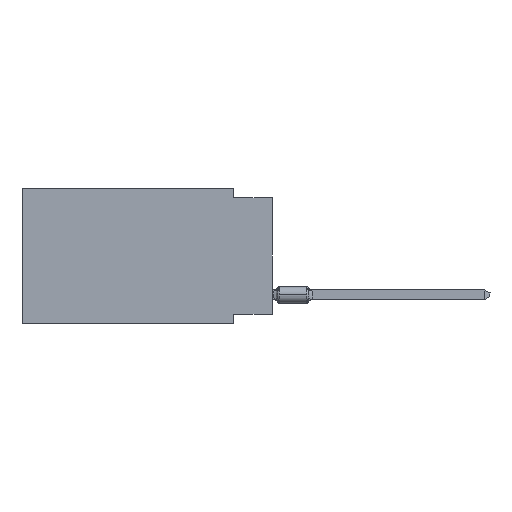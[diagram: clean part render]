
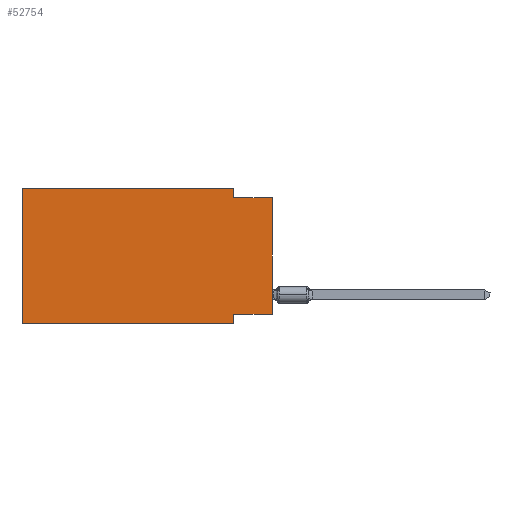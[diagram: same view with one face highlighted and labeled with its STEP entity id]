
A CAD part, left-side view. The second image highlights one B-rep face of the part: STEP entity #52754.
In plain terms, the highlighted planar face has unit normal (-1, 0, 0).
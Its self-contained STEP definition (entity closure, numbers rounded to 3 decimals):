
#568 = PLANE ( 'NONE',  #59043 ) ;
#885 = CARTESIAN_POINT ( 'NONE',  ( 0., 16.383, -8.89 ) ) ;
#1793 = DIRECTION ( 'NONE',  ( 0., 0., 1. ) ) ;
#2591 = CARTESIAN_POINT ( 'NONE',  ( 0., 2.54, -8.89 ) ) ;
#4227 = VERTEX_POINT ( 'NONE', #55370 ) ;
#4961 = CARTESIAN_POINT ( 'NONE',  ( 0., 0., -0.635 ) ) ;
#8224 = VECTOR ( 'NONE', #14936, 1000. ) ;
#10448 = LINE ( 'NONE', #34493, #51431 ) ;
#10690 = CARTESIAN_POINT ( 'NONE',  ( 0., 16.383, 0. ) ) ;
#11004 = VECTOR ( 'NONE', #1793, 1000. ) ;
#12177 = EDGE_CURVE ( 'NONE', #58907, #16448, #28717, .T. ) ;
#13767 = EDGE_CURVE ( 'NONE', #4227, #40827, #45387, .T. ) ;
#14033 = DIRECTION ( 'NONE',  ( 0., 0., -1. ) ) ;
#14936 = DIRECTION ( 'NONE',  ( 0., 1., 0. ) ) ;
#14949 = CARTESIAN_POINT ( 'NONE',  ( 0., 2.54, 0. ) ) ;
#15341 = EDGE_CURVE ( 'NONE', #35343, #16448, #57782, .T. ) ;
#16448 = VERTEX_POINT ( 'NONE', #4961 ) ;
#17211 = VERTEX_POINT ( 'NONE', #45778 ) ;
#18055 = ORIENTED_EDGE ( 'NONE', *, *, #25695, .F. ) ;
#20013 = VERTEX_POINT ( 'NONE', #10690 ) ;
#20449 = EDGE_LOOP ( 'NONE', ( #37459, #60444, #48436, #32620, #18055, #57352, #57975, #26336 ) ) ;
#21483 = LINE ( 'NONE', #26184, #60625 ) ;
#21529 = VECTOR ( 'NONE', #24655, 1000. ) ;
#24655 = DIRECTION ( 'NONE',  ( 0., -1., 0. ) ) ;
#25243 = DIRECTION ( 'NONE',  ( 1., 0., 0. ) ) ;
#25494 = CARTESIAN_POINT ( 'NONE',  ( 0., 16.383, -8.89 ) ) ;
#25695 = EDGE_CURVE ( 'NONE', #33477, #20013, #10448, .T. ) ;
#26184 = CARTESIAN_POINT ( 'NONE',  ( 0., 16.383, 0. ) ) ;
#26336 = ORIENTED_EDGE ( 'NONE', *, *, #53541, .F. ) ;
#27827 = EDGE_CURVE ( 'NONE', #17211, #58907, #47752, .T. ) ;
#28717 = LINE ( 'NONE', #38415, #21529 ) ;
#32620 = ORIENTED_EDGE ( 'NONE', *, *, #35200, .F. ) ;
#33477 = VERTEX_POINT ( 'NONE', #885 ) ;
#34493 = CARTESIAN_POINT ( 'NONE',  ( 0., 16.383, 0. ) ) ;
#34623 = CARTESIAN_POINT ( 'NONE',  ( 0., 0., -8.255 ) ) ;
#35189 = LINE ( 'NONE', #25494, #42277 ) ;
#35200 = EDGE_CURVE ( 'NONE', #20013, #17211, #21483, .T. ) ;
#35343 = VERTEX_POINT ( 'NONE', #37402 ) ;
#35699 = DIRECTION ( 'NONE',  ( 0., 0., -1. ) ) ;
#37402 = CARTESIAN_POINT ( 'NONE',  ( 0., 0., -8.255 ) ) ;
#37459 = ORIENTED_EDGE ( 'NONE', *, *, #15341, .T. ) ;
#38415 = CARTESIAN_POINT ( 'NONE',  ( 0., 0., -0.635 ) ) ;
#39320 = FACE_OUTER_BOUND ( 'NONE', #20449, .T. ) ;
#39983 = EDGE_CURVE ( 'NONE', #33477, #40827, #35189, .T. ) ;
#40613 = CARTESIAN_POINT ( 'NONE',  ( 0., 2.54, -0.635 ) ) ;
#40827 = VERTEX_POINT ( 'NONE', #52859 ) ;
#42277 = VECTOR ( 'NONE', #53955, 1000. ) ;
#43492 = VECTOR ( 'NONE', #14033, 1000. ) ;
#44634 = CARTESIAN_POINT ( 'NONE',  ( 0., 16.383, 0. ) ) ;
#45387 = LINE ( 'NONE', #2591, #61706 ) ;
#45550 = DIRECTION ( 'NONE',  ( 0., -1., 0. ) ) ;
#45778 = CARTESIAN_POINT ( 'NONE',  ( 0., 2.54, 0. ) ) ;
#47752 = LINE ( 'NONE', #14949, #43492 ) ;
#48238 = DIRECTION ( 'NONE',  ( 0., 0., 1. ) ) ;
#48436 = ORIENTED_EDGE ( 'NONE', *, *, #27827, .F. ) ;
#48687 = DIRECTION ( 'NONE',  ( 0., 0., -1. ) ) ;
#51431 = VECTOR ( 'NONE', #48238, 1000. ) ;
#52754 = ADVANCED_FACE ( 'NONE', ( #39320 ), #568, .F. ) ;
#52859 = CARTESIAN_POINT ( 'NONE',  ( 0., 2.54, -8.89 ) ) ;
#53111 = CARTESIAN_POINT ( 'NONE',  ( 0., 0., 0. ) ) ;
#53541 = EDGE_CURVE ( 'NONE', #35343, #4227, #58058, .T. ) ;
#53955 = DIRECTION ( 'NONE',  ( 0., -1., 0. ) ) ;
#55370 = CARTESIAN_POINT ( 'NONE',  ( 0., 2.54, -8.255 ) ) ;
#57352 = ORIENTED_EDGE ( 'NONE', *, *, #39983, .T. ) ;
#57782 = LINE ( 'NONE', #53111, #11004 ) ;
#57975 = ORIENTED_EDGE ( 'NONE', *, *, #13767, .F. ) ;
#58058 = LINE ( 'NONE', #34623, #8224 ) ;
#58907 = VERTEX_POINT ( 'NONE', #40613 ) ;
#59043 = AXIS2_PLACEMENT_3D ( 'NONE', #44634, #25243, #48687 ) ;
#60444 = ORIENTED_EDGE ( 'NONE', *, *, #12177, .F. ) ;
#60625 = VECTOR ( 'NONE', #45550, 1000. ) ;
#61706 = VECTOR ( 'NONE', #35699, 1000. ) ;
